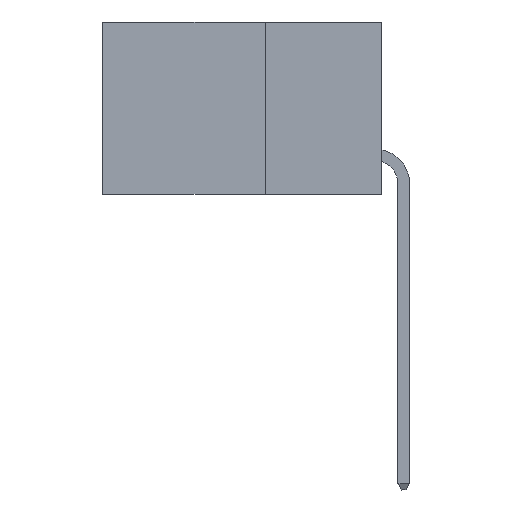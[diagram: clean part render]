
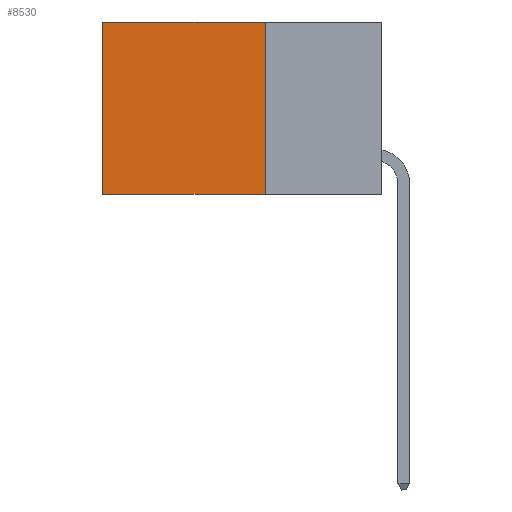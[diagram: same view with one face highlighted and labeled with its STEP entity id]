
A CAD part, left-side view. The second image highlights one B-rep face of the part: STEP entity #8530.
In plain terms, the highlighted planar face has unit normal (-1, 0, 0).
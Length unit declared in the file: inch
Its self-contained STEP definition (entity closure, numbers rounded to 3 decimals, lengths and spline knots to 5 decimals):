
#169 = AXIS2_PLACEMENT_3D ( 'NONE', #7980, #8747, #4051 ) ;
#546 = VECTOR ( 'NONE', #2512, 39.37008 ) ;
#691 = VERTEX_POINT ( 'NONE', #2311 ) ;
#1210 = CARTESIAN_POINT ( 'NONE',  ( 0.2875, 0.6, 0. ) ) ;
#1364 = EDGE_CURVE ( 'NONE', #1960, #7360, #9536, .T. ) ;
#1754 = CARTESIAN_POINT ( 'NONE',  ( 0.2875, 0.25, 0. ) ) ;
#1960 = VERTEX_POINT ( 'NONE', #8415 ) ;
#2090 = ORIENTED_EDGE ( 'NONE', *, *, #8785, .T. ) ;
#2211 = EDGE_CURVE ( 'NONE', #9733, #7360, #7581, .T. ) ;
#2311 = CARTESIAN_POINT ( 'NONE',  ( 0.2875, 0.25, 0. ) ) ;
#2512 = DIRECTION ( 'NONE',  ( 0., 0., -1. ) ) ;
#2604 = DIRECTION ( 'NONE',  ( 0., 0., -1. ) ) ;
#3027 = EDGE_LOOP ( 'NONE', ( #6058, #8108, #10255, #2090 ) ) ;
#3503 = CARTESIAN_POINT ( 'NONE',  ( 0.2875, 0.6, -0.37 ) ) ;
#4051 = DIRECTION ( 'NONE',  ( 0., 0., -1. ) ) ;
#4106 = CARTESIAN_POINT ( 'NONE',  ( 0.2875, 0.25, -0.37 ) ) ;
#4113 = VECTOR ( 'NONE', #7550, 39.37008 ) ;
#4332 = DIRECTION ( 'NONE',  ( 0., 1., 0. ) ) ;
#6058 = ORIENTED_EDGE ( 'NONE', *, *, #1364, .T. ) ;
#6125 = VECTOR ( 'NONE', #4332, 39.37008 ) ;
#6245 = LINE ( 'NONE', #1754, #4113 ) ;
#7232 = CARTESIAN_POINT ( 'NONE',  ( 0.2875, 0.25, -0.37 ) ) ;
#7250 = PLANE ( 'NONE',  #169 ) ;
#7360 = VERTEX_POINT ( 'NONE', #3503 ) ;
#7550 = DIRECTION ( 'NONE',  ( 0., 1., 0. ) ) ;
#7581 = LINE ( 'NONE', #4106, #6125 ) ;
#7980 = CARTESIAN_POINT ( 'NONE',  ( 0.2875, 0.25, 0. ) ) ;
#8108 = ORIENTED_EDGE ( 'NONE', *, *, #2211, .F. ) ;
#8415 = CARTESIAN_POINT ( 'NONE',  ( 0.2875, 0.6, 0. ) ) ;
#8530 = ADVANCED_FACE ( 'NONE', ( #8867 ), #7250, .F. ) ;
#8655 = VECTOR ( 'NONE', #2604, 39.37008 ) ;
#8747 = DIRECTION ( 'NONE',  ( 1., 0., 0. ) ) ;
#8785 = EDGE_CURVE ( 'NONE', #691, #1960, #6245, .T. ) ;
#8867 = FACE_OUTER_BOUND ( 'NONE', #3027, .T. ) ;
#9329 = EDGE_CURVE ( 'NONE', #691, #9733, #9388, .T. ) ;
#9388 = LINE ( 'NONE', #10358, #546 ) ;
#9536 = LINE ( 'NONE', #1210, #8655 ) ;
#9733 = VERTEX_POINT ( 'NONE', #7232 ) ;
#10255 = ORIENTED_EDGE ( 'NONE', *, *, #9329, .F. ) ;
#10358 = CARTESIAN_POINT ( 'NONE',  ( 0.2875, 0.25, 0. ) ) ;
